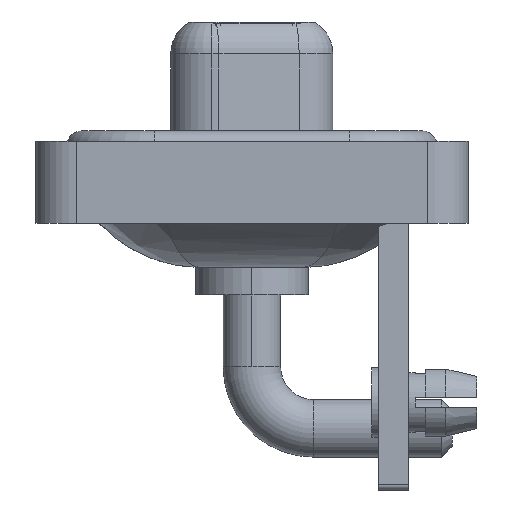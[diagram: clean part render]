
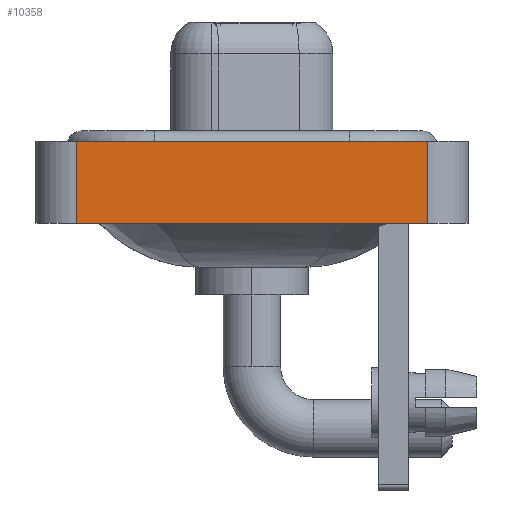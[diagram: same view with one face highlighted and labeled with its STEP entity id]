
A CAD part, left-side view. The second image highlights one B-rep face of the part: STEP entity #10358.
In plain terms, the highlighted planar face has unit normal (-1, 0, 0).
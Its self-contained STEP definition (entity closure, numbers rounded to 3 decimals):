
#7 = CARTESIAN_POINT ( 'NONE',  ( -7.25, 8.55, 0.4 ) ) ;
#852 = ORIENTED_EDGE ( 'NONE', *, *, #2954, .T. ) ;
#1367 = DIRECTION ( 'NONE',  ( -1., 0., 0. ) ) ;
#1487 = DIRECTION ( 'NONE',  ( 0., 0., 1. ) ) ;
#1653 = VERTEX_POINT ( 'NONE', #5859 ) ;
#2101 = CARTESIAN_POINT ( 'NONE',  ( -7.25, -8.55, -3.6 ) ) ;
#2954 = EDGE_CURVE ( 'NONE', #9669, #4038, #5420, .T. ) ;
#3217 = VECTOR ( 'NONE', #15815, 1000. ) ;
#4038 = VERTEX_POINT ( 'NONE', #2101 ) ;
#4319 = PLANE ( 'NONE',  #8457 ) ;
#4410 = CARTESIAN_POINT ( 'NONE',  ( -7.25, -8.55, -3.6 ) ) ;
#5233 = ORIENTED_EDGE ( 'NONE', *, *, #11257, .F. ) ;
#5420 = LINE ( 'NONE', #13727, #9727 ) ;
#5556 = LINE ( 'NONE', #8786, #3217 ) ;
#5859 = CARTESIAN_POINT ( 'NONE',  ( -7.25, -8.55, 0.4 ) ) ;
#6711 = DIRECTION ( 'NONE',  ( 0., -1., 0. ) ) ;
#7860 = VECTOR ( 'NONE', #11328, 1000. ) ;
#8380 = FACE_OUTER_BOUND ( 'NONE', #9008, .T. ) ;
#8457 = AXIS2_PLACEMENT_3D ( 'NONE', #4410, #1367, #12527 ) ;
#8786 = CARTESIAN_POINT ( 'NONE',  ( -7.25, -8.55, -3.6 ) ) ;
#9008 = EDGE_LOOP ( 'NONE', ( #15084, #10750, #5233, #852 ) ) ;
#9669 = VERTEX_POINT ( 'NONE', #12005 ) ;
#9727 = VECTOR ( 'NONE', #6711, 1000. ) ;
#10150 = VECTOR ( 'NONE', #1487, 1000. ) ;
#10347 = EDGE_CURVE ( 'NONE', #12178, #1653, #17078, .T. ) ;
#10358 = ADVANCED_FACE ( 'NONE', ( #8380 ), #4319, .T. ) ;
#10750 = ORIENTED_EDGE ( 'NONE', *, *, #10347, .F. ) ;
#11257 = EDGE_CURVE ( 'NONE', #9669, #12178, #14325, .T. ) ;
#11328 = DIRECTION ( 'NONE',  ( 0., -1., 0. ) ) ;
#12005 = CARTESIAN_POINT ( 'NONE',  ( -7.25, 8.55, -3.6 ) ) ;
#12178 = VERTEX_POINT ( 'NONE', #7 ) ;
#12527 = DIRECTION ( 'NONE',  ( 0., 0., 1. ) ) ;
#13727 = CARTESIAN_POINT ( 'NONE',  ( -7.25, -8.55, -3.6 ) ) ;
#14298 = CARTESIAN_POINT ( 'NONE',  ( -7.25, -8.55, 0.4 ) ) ;
#14325 = LINE ( 'NONE', #15622, #10150 ) ;
#15084 = ORIENTED_EDGE ( 'NONE', *, *, #16316, .T. ) ;
#15622 = CARTESIAN_POINT ( 'NONE',  ( -7.25, 8.55, -3.6 ) ) ;
#15815 = DIRECTION ( 'NONE',  ( 0., 0., 1. ) ) ;
#16316 = EDGE_CURVE ( 'NONE', #4038, #1653, #5556, .T. ) ;
#17078 = LINE ( 'NONE', #14298, #7860 ) ;
